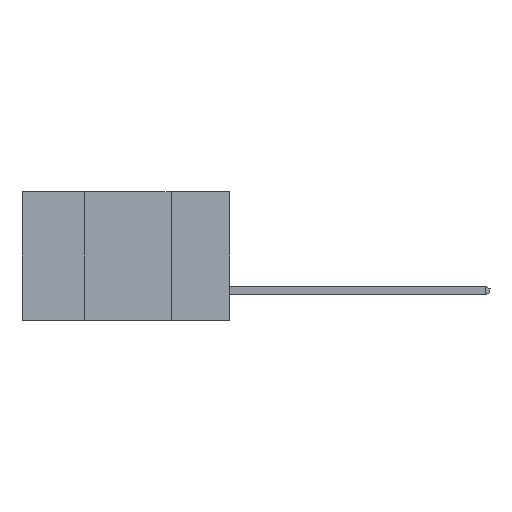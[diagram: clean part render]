
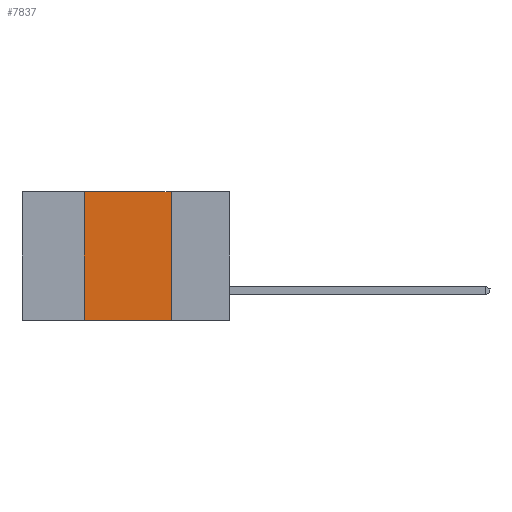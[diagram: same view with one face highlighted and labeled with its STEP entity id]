
A CAD part, left-side view. The second image highlights one B-rep face of the part: STEP entity #7837.
In plain terms, the highlighted planar face has unit normal (-1, 0, 0).
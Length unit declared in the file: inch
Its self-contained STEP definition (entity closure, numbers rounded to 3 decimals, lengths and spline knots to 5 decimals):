
#462 = VECTOR ( 'NONE', #6055, 39.37008 ) ;
#558 = DIRECTION ( 'NONE',  ( 1., 0., 0. ) ) ;
#627 = CARTESIAN_POINT ( 'NONE',  ( 0., 0.6, 0. ) ) ;
#752 = EDGE_CURVE ( 'NONE', #10323, #10992, #11702, .T. ) ;
#1411 = CARTESIAN_POINT ( 'NONE',  ( 0., 0.17, 0. ) ) ;
#1538 = DIRECTION ( 'NONE',  ( 0., 0., -1. ) ) ;
#1761 = EDGE_CURVE ( 'NONE', #10992, #9295, #13201, .T. ) ;
#1844 = CARTESIAN_POINT ( 'NONE',  ( 0., 0.42, -0.37 ) ) ;
#2705 = CARTESIAN_POINT ( 'NONE',  ( 0., 0.6, -0.37 ) ) ;
#2838 = EDGE_LOOP ( 'NONE', ( #8544, #8009, #5280, #9184 ) ) ;
#2878 = VECTOR ( 'NONE', #2991, 39.37008 ) ;
#2991 = DIRECTION ( 'NONE',  ( 0., 0., 1. ) ) ;
#3795 = LINE ( 'NONE', #5855, #3892 ) ;
#3892 = VECTOR ( 'NONE', #10159, 39.37008 ) ;
#5280 = ORIENTED_EDGE ( 'NONE', *, *, #752, .F. ) ;
#5855 = CARTESIAN_POINT ( 'NONE',  ( 0., 0.17, -0.37 ) ) ;
#6055 = DIRECTION ( 'NONE',  ( 0., -1., 0. ) ) ;
#6833 = CARTESIAN_POINT ( 'NONE',  ( 0., 0.6, 0. ) ) ;
#7026 = FACE_OUTER_BOUND ( 'NONE', #2838, .T. ) ;
#7352 = EDGE_CURVE ( 'NONE', #10323, #8631, #10212, .T. ) ;
#7837 = ADVANCED_FACE ( 'NONE', ( #7026 ), #8062, .F. ) ;
#8009 = ORIENTED_EDGE ( 'NONE', *, *, #1761, .F. ) ;
#8062 = PLANE ( 'NONE',  #10667 ) ;
#8191 = EDGE_CURVE ( 'NONE', #9295, #8631, #3795, .T. ) ;
#8544 = ORIENTED_EDGE ( 'NONE', *, *, #8191, .F. ) ;
#8628 = VECTOR ( 'NONE', #12085, 39.37008 ) ;
#8631 = VERTEX_POINT ( 'NONE', #11011 ) ;
#8661 = CARTESIAN_POINT ( 'NONE',  ( 0., 0.42, 0. ) ) ;
#9184 = ORIENTED_EDGE ( 'NONE', *, *, #7352, .T. ) ;
#9295 = VERTEX_POINT ( 'NONE', #1411 ) ;
#10159 = DIRECTION ( 'NONE',  ( 0., 0., -1. ) ) ;
#10212 = LINE ( 'NONE', #2705, #462 ) ;
#10323 = VERTEX_POINT ( 'NONE', #11100 ) ;
#10667 = AXIS2_PLACEMENT_3D ( 'NONE', #627, #558, #1538 ) ;
#10992 = VERTEX_POINT ( 'NONE', #8661 ) ;
#11011 = CARTESIAN_POINT ( 'NONE',  ( 0., 0.17, -0.37 ) ) ;
#11100 = CARTESIAN_POINT ( 'NONE',  ( 0., 0.42, -0.37 ) ) ;
#11702 = LINE ( 'NONE', #1844, #2878 ) ;
#12085 = DIRECTION ( 'NONE',  ( 0., -1., 0. ) ) ;
#13201 = LINE ( 'NONE', #6833, #8628 ) ;
